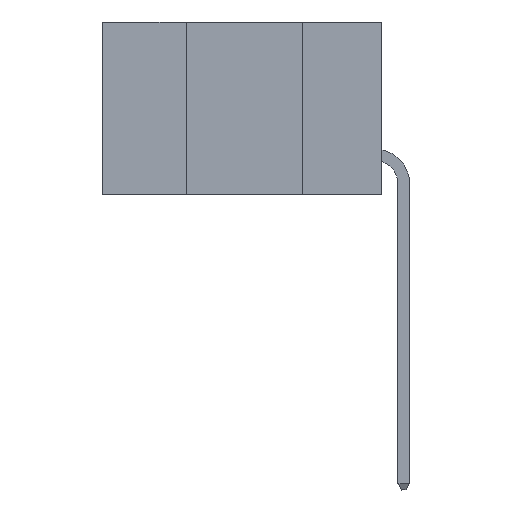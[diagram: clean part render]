
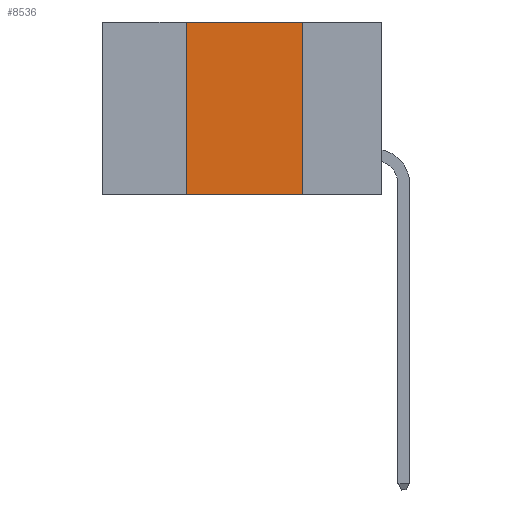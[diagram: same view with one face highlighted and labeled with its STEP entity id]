
A CAD part, left-side view. The second image highlights one B-rep face of the part: STEP entity #8536.
In plain terms, the highlighted planar face has unit normal (-1, 0, 0).
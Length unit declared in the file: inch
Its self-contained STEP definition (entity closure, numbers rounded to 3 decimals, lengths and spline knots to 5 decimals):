
#369 = FACE_OUTER_BOUND ( 'NONE', #25866, .T. ) ;
#3266 = CARTESIAN_POINT ( 'NONE',  ( 0., 0.17, 0. ) ) ;
#3507 = DIRECTION ( 'NONE',  ( 1., 0., 0. ) ) ;
#3824 = VECTOR ( 'NONE', #38123, 39.37008 ) ;
#5444 = VECTOR ( 'NONE', #38035, 39.37008 ) ;
#5774 = ORIENTED_EDGE ( 'NONE', *, *, #19929, .T. ) ;
#6501 = EDGE_CURVE ( 'NONE', #15846, #7452, #25447, .T. ) ;
#6728 = PLANE ( 'NONE',  #31964 ) ;
#7452 = VERTEX_POINT ( 'NONE', #29636 ) ;
#8536 = ADVANCED_FACE ( 'NONE', ( #369 ), #6728, .F. ) ;
#10333 = CARTESIAN_POINT ( 'NONE',  ( 0., 0.6, 0. ) ) ;
#11121 = LINE ( 'NONE', #32172, #13539 ) ;
#13148 = ORIENTED_EDGE ( 'NONE', *, *, #17966, .F. ) ;
#13539 = VECTOR ( 'NONE', #20413, 39.37008 ) ;
#13587 = LINE ( 'NONE', #19371, #5444 ) ;
#14272 = DIRECTION ( 'NONE',  ( 0., -1., 0. ) ) ;
#15807 = CARTESIAN_POINT ( 'NONE',  ( 0., 0.42, -0.37 ) ) ;
#15846 = VERTEX_POINT ( 'NONE', #32228 ) ;
#16760 = VECTOR ( 'NONE', #14272, 39.37008 ) ;
#17966 = EDGE_CURVE ( 'NONE', #27777, #15846, #22991, .T. ) ;
#19371 = CARTESIAN_POINT ( 'NONE',  ( 0., 0.6, -0.37 ) ) ;
#19929 = EDGE_CURVE ( 'NONE', #34643, #7452, #13587, .T. ) ;
#20413 = DIRECTION ( 'NONE',  ( 0., 0., 1. ) ) ;
#21804 = ORIENTED_EDGE ( 'NONE', *, *, #23370, .F. ) ;
#22991 = LINE ( 'NONE', #10333, #16760 ) ;
#23370 = EDGE_CURVE ( 'NONE', #34643, #27777, #11121, .T. ) ;
#24367 = ORIENTED_EDGE ( 'NONE', *, *, #6501, .F. ) ;
#25447 = LINE ( 'NONE', #3266, #3824 ) ;
#25866 = EDGE_LOOP ( 'NONE', ( #24367, #13148, #21804, #5774 ) ) ;
#27777 = VERTEX_POINT ( 'NONE', #35789 ) ;
#29636 = CARTESIAN_POINT ( 'NONE',  ( 0., 0.17, -0.37 ) ) ;
#31964 = AXIS2_PLACEMENT_3D ( 'NONE', #37168, #3507, #35116 ) ;
#32172 = CARTESIAN_POINT ( 'NONE',  ( 0., 0.42, 0. ) ) ;
#32228 = CARTESIAN_POINT ( 'NONE',  ( 0., 0.17, 0. ) ) ;
#34643 = VERTEX_POINT ( 'NONE', #15807 ) ;
#35116 = DIRECTION ( 'NONE',  ( 0., 0., -1. ) ) ;
#35789 = CARTESIAN_POINT ( 'NONE',  ( 0., 0.42, 0. ) ) ;
#37168 = CARTESIAN_POINT ( 'NONE',  ( 0., 0.6, 0. ) ) ;
#38035 = DIRECTION ( 'NONE',  ( 0., -1., 0. ) ) ;
#38123 = DIRECTION ( 'NONE',  ( 0., 0., -1. ) ) ;
